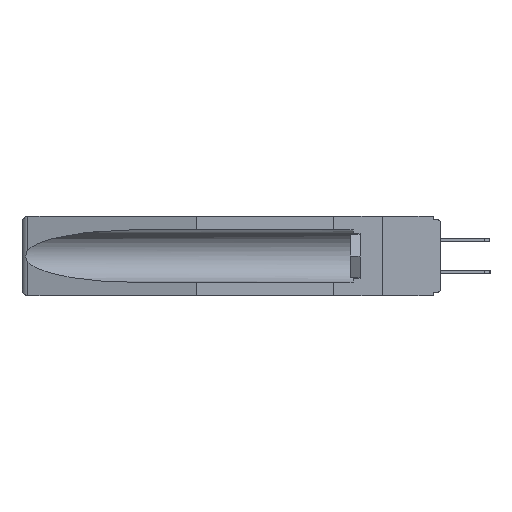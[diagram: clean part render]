
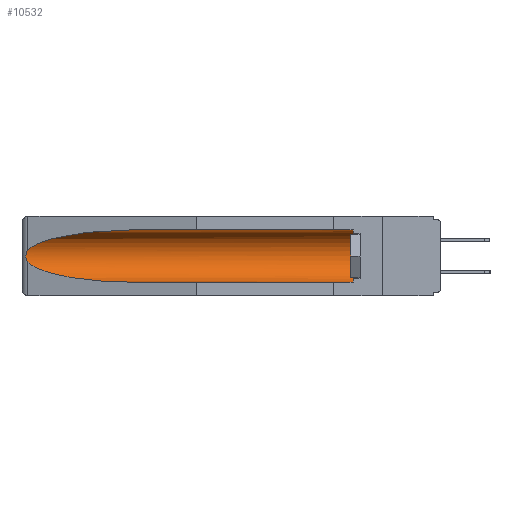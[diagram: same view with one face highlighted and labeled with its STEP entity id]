
A CAD part, left-side view. The second image highlights one B-rep face of the part: STEP entity #10532.
In plain terms, the highlighted cylindrical face has radius 2.857 mm (diameter 5.715 mm), a partial arc.
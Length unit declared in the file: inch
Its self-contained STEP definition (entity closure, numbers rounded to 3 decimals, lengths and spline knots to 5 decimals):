
#108 = CARTESIAN_POINT ( 'NONE',  ( 0.26537, 1.52718, -0.14972 ) ) ;
#811 = VECTOR ( 'NONE', #5669, 39.37008 ) ;
#1431 = CARTESIAN_POINT ( 'NONE',  ( 0.26537, 1.52718, -0.19328 ) ) ;
#2462 = VERTEX_POINT ( 'NONE', #5752 ) ;
#3109 = VERTEX_POINT ( 'NONE', #7768 ) ;
#3690 = VERTEX_POINT ( 'NONE', #108 ) ;
#3761 = CARTESIAN_POINT ( 'NONE',  ( 0.26537, 1.52718, -0.14972 ) ) ;
#3789 = VECTOR ( 'NONE', #7808, 39.37008 ) ;
#4249 = CARTESIAN_POINT ( 'NONE',  ( 0.2673, 1.5327, -0.16383 ) ) ;
#4341 =( BOUNDED_CURVE ( )  B_SPLINE_CURVE ( 3, ( #20791, #12505, #10210, #3761 ),
 .UNSPECIFIED., .F., .F. ) 
 B_SPLINE_CURVE_WITH_KNOTS ( ( 4, 4 ),
 ( 4.71239, 6.08839 ),
 .UNSPECIFIED. ) 
 CURVE ( )  GEOMETRIC_REPRESENTATION_ITEM ( )  RATIONAL_B_SPLINE_CURVE ( ( 1., 0.848, 0.848, 1. ) ) 
 REPRESENTATION_ITEM ( '' )  );
#5525 = LINE ( 'NONE', #9965, #811 ) ;
#5555 =( BOUNDED_CURVE ( )  B_SPLINE_CURVE ( 3, ( #1431, #9957, #24791, #7793 ),
 .UNSPECIFIED., .F., .T. ) 
 B_SPLINE_CURVE_WITH_KNOTS ( ( 4, 4 ),
 ( 0.1948, 1.5708 ),
 .UNSPECIFIED. ) 
 CURVE ( )  GEOMETRIC_REPRESENTATION_ITEM ( )  RATIONAL_B_SPLINE_CURVE ( ( 1., 0.848, 0.848, 1. ) ) 
 REPRESENTATION_ITEM ( '' )  );
#5560 = ORIENTED_EDGE ( 'NONE', *, *, #14536, .T. ) ;
#5579 = ORIENTED_EDGE ( 'NONE', *, *, #10142, .T. ) ;
#5638 = VERTEX_POINT ( 'NONE', #14356 ) ;
#5669 = DIRECTION ( 'NONE',  ( 0., 1., 0. ) ) ;
#5752 = CARTESIAN_POINT ( 'NONE',  ( 0.155, 1.07973, -0.059 ) ) ;
#5938 = DIRECTION ( 'NONE',  ( 0., -1., 0. ) ) ;
#6560 = CARTESIAN_POINT ( 'NONE',  ( 0.2675, 1.53308, -0.16763 ) ) ;
#6994 = DIRECTION ( 'NONE',  ( 0., 0., 1. ) ) ;
#7629 = ORIENTED_EDGE ( 'NONE', *, *, #15823, .T. ) ;
#7768 = CARTESIAN_POINT ( 'NONE',  ( 0.155, 0.126, -0.284 ) ) ;
#7793 = CARTESIAN_POINT ( 'NONE',  ( 0.155, 1.07973, -0.284 ) ) ;
#7808 = DIRECTION ( 'NONE',  ( 0., 1., 0. ) ) ;
#7909 = CARTESIAN_POINT ( 'NONE',  ( 0.155, -0.30754, -0.284 ) ) ;
#8293 = EDGE_LOOP ( 'NONE', ( #12648, #17410, #5560, #27561, #5579, #7629 ) ) ;
#8336 = EDGE_CURVE ( 'NONE', #3109, #5638, #9484, .T. ) ;
#8510 = CYLINDRICAL_SURFACE ( 'NONE', #23340, 0.1125 ) ;
#8643 = CARTESIAN_POINT ( 'NONE',  ( 0.26654, 1.53092, -0.15636 ) ) ;
#9484 = LINE ( 'NONE', #7909, #3789 ) ;
#9693 = CIRCLE ( 'NONE', #23512, 0.1125 ) ;
#9957 = CARTESIAN_POINT ( 'NONE',  ( 0.25451, 1.48313, -0.24835 ) ) ;
#9965 = CARTESIAN_POINT ( 'NONE',  ( 0.155, -0.30754, -0.059 ) ) ;
#10142 = EDGE_CURVE ( 'NONE', #3109, #19387, #9693, .T. ) ;
#10210 = CARTESIAN_POINT ( 'NONE',  ( 0.25451, 1.48313, -0.09465 ) ) ;
#10532 = ADVANCED_FACE ( 'NONE', ( #22461 ), #8510, .F. ) ;
#10579 = DIRECTION ( 'NONE',  ( 0., 1., 0. ) ) ;
#12505 = CARTESIAN_POINT ( 'NONE',  ( 0.21114, 1.30732, -0.059 ) ) ;
#12648 = ORIENTED_EDGE ( 'NONE', *, *, #20266, .T. ) ;
#12716 = CARTESIAN_POINT ( 'NONE',  ( 0.26597, 1.52961, -0.15275 ) ) ;
#12893 = CARTESIAN_POINT ( 'NONE',  ( 0.2675, 1.53308, -0.17534 ) ) ;
#14356 = CARTESIAN_POINT ( 'NONE',  ( 0.155, 1.07973, -0.284 ) ) ;
#14536 = EDGE_CURVE ( 'NONE', #21756, #5638, #5555, .T. ) ;
#14735 = CARTESIAN_POINT ( 'NONE',  ( 0.155, -0.30754, -0.1715 ) ) ;
#15067 = CARTESIAN_POINT ( 'NONE',  ( 0.26537, 1.52718, -0.19328 ) ) ;
#15455 = CARTESIAN_POINT ( 'NONE',  ( 0.155, 0.126, -0.059 ) ) ;
#15823 = EDGE_CURVE ( 'NONE', #19387, #2462, #5525, .T. ) ;
#16834 = CARTESIAN_POINT ( 'NONE',  ( 0.26597, 1.5296, -0.19026 ) ) ;
#17410 = ORIENTED_EDGE ( 'NONE', *, *, #23308, .T. ) ;
#18761 = CARTESIAN_POINT ( 'NONE',  ( 0.155, 0.126, -0.1715 ) ) ;
#19132 = CARTESIAN_POINT ( 'NONE',  ( 0.2673, 1.53269, -0.17917 ) ) ;
#19387 = VERTEX_POINT ( 'NONE', #15455 ) ;
#20266 = EDGE_CURVE ( 'NONE', #2462, #3690, #4341, .T. ) ;
#20791 = CARTESIAN_POINT ( 'NONE',  ( 0.155, 1.07973, -0.059 ) ) ;
#20814 = DIRECTION ( 'NONE',  ( 0., 0., 1. ) ) ;
#21756 = VERTEX_POINT ( 'NONE', #22483 ) ;
#22461 = FACE_OUTER_BOUND ( 'NONE', #8293, .T. ) ;
#22483 = CARTESIAN_POINT ( 'NONE',  ( 0.26537, 1.52718, -0.19328 ) ) ;
#23213 = CARTESIAN_POINT ( 'NONE',  ( 0.26655, 1.53094, -0.18657 ) ) ;
#23308 = EDGE_CURVE ( 'NONE', #3690, #21756, #26204, .T. ) ;
#23340 = AXIS2_PLACEMENT_3D ( 'NONE', #14735, #10579, #6994 ) ;
#23512 = AXIS2_PLACEMENT_3D ( 'NONE', #18761, #5938, #20814 ) ;
#24791 = CARTESIAN_POINT ( 'NONE',  ( 0.21114, 1.30732, -0.284 ) ) ;
#25453 = CARTESIAN_POINT ( 'NONE',  ( 0.26537, 1.52718, -0.14972 ) ) ;
#26204 = B_SPLINE_CURVE_WITH_KNOTS ( 'NONE', 3,
 ( #25453, #12716, #8643, #4249, #6560, #12893, #19132, #23213, #16834, #15067 ),
 .UNSPECIFIED., .F., .F.,
 ( 4, 2, 2, 2, 4 ),
 ( 0., 0.00029, 0.00058, 0.00087, 0.00117 ),
 .UNSPECIFIED. ) ;
#27561 = ORIENTED_EDGE ( 'NONE', *, *, #8336, .F. ) ;
